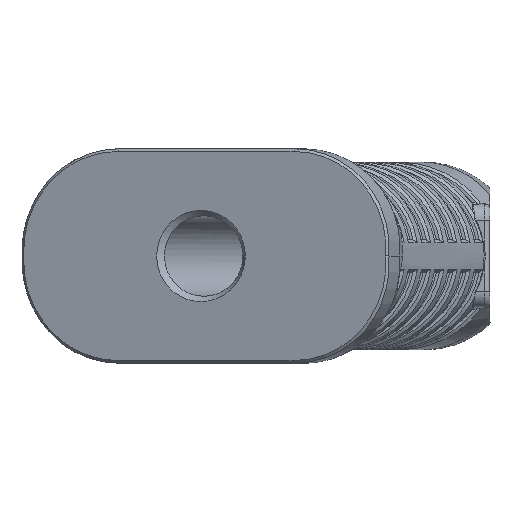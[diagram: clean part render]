
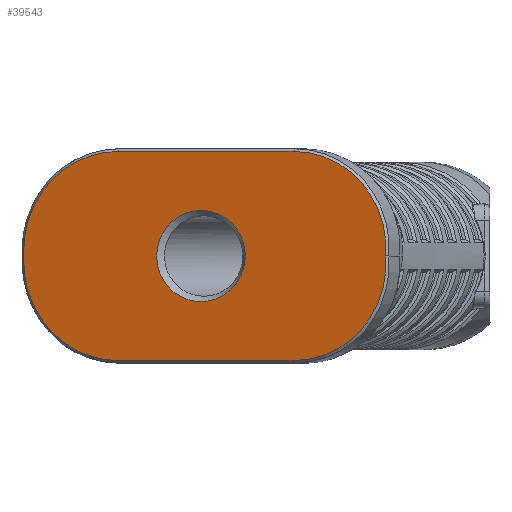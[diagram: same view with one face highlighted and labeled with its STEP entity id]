
A CAD part, front view. The second image highlights one B-rep face of the part: STEP entity #39543.
In plain terms, the highlighted planar face has unit normal (-0.307, -0.952, 0).
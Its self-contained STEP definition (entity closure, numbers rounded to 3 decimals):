
#153 = CARTESIAN_POINT ( 'NONE',  ( -220.334, -103.035, 0. ) ) ;
#214 = CARTESIAN_POINT ( 'NONE',  ( -220.334, -103.035, 4.858 ) ) ;
#435 = CARTESIAN_POINT ( 'NONE',  ( -169.904, -119.324, 2.5 ) ) ;
#636 = AXIS2_PLACEMENT_3D ( 'NONE', #8100, #1470, #26456 ) ;
#975 = VERTEX_POINT ( 'NONE', #10771 ) ;
#1265 = DIRECTION ( 'NONE',  ( -0.952, 0.307, 0. ) ) ;
#1470 = DIRECTION ( 'NONE',  ( 0.307, 0.952, 0. ) ) ;
#2087 = PLANE ( 'NONE',  #22072 ) ;
#2215 = CARTESIAN_POINT ( 'NONE',  ( -184.975, -114.456, 1. ) ) ;
#2891 = ORIENTED_EDGE ( 'NONE', *, *, #38587, .F. ) ;
#3178 = CARTESIAN_POINT ( 'NONE',  ( -217.258, -104.029, 12.827 ) ) ;
#3328 = CARTESIAN_POINT ( 'NONE',  ( -219.695, -103.242, 7.717 ) ) ;
#3631 = CARTESIAN_POINT ( 'NONE',  ( -185.365, -114.33, -7.569 ) ) ;
#4032 = CARTESIAN_POINT ( 'NONE',  ( -182.305, -115.318, 8.167 ) ) ;
#4284 = CARTESIAN_POINT ( 'NONE',  ( -213.297, -105.308, -14.8 ) ) ;
#4331 = ORIENTED_EDGE ( 'NONE', *, *, #37915, .F. ) ;
#4962 = DIRECTION ( 'NONE',  ( 0.952, -0.307, 0. ) ) ;
#5083 = CARTESIAN_POINT ( 'NONE',  ( -220.334, -103.035, 2. ) ) ;
#5459 = CARTESIAN_POINT ( 'NONE',  ( -220.334, -103.035, 0.5 ) ) ;
#5884 = CARTESIAN_POINT ( 'NONE',  ( -220.334, -103.035, 2. ) ) ;
#5949 = CARTESIAN_POINT ( 'NONE',  ( -202.734, -108.72, 20.5 ) ) ;
#6022 = CARTESIAN_POINT ( 'NONE',  ( -213.297, -105.308, 16.8 ) ) ;
#6035 = DIRECTION ( 'NONE',  ( 0.307, 0.952, 0. ) ) ;
#6374 = CARTESIAN_POINT ( 'NONE',  ( -215.784, -104.505, -12.839 ) ) ;
#6432 = CARTESIAN_POINT ( 'NONE',  ( -215.474, -104.605, 15.085 ) ) ;
#6771 = CARTESIAN_POINT ( 'NONE',  ( -195.511, -111.053, 1. ) ) ;
#6895 = CARTESIAN_POINT ( 'NONE',  ( -192.57, -112.003, -5.881 ) ) ;
#7104 = B_SPLINE_CURVE_WITH_KNOTS ( 'NONE', 3,
 ( #5884, #214, #3328, #3178, #6432, #6022 ),
 .UNSPECIFIED., .F., .F.,
 ( 4, 2, 4 ),
 ( 0., 0.5, 1. ),
 .UNSPECIFIED. ) ;
#7576 = CARTESIAN_POINT ( 'NONE',  ( -169.904, -119.324, -18.5 ) ) ;
#8100 = CARTESIAN_POINT ( 'NONE',  ( -202.734, -108.72, 2. ) ) ;
#8741 = DIRECTION ( 'NONE',  ( 0.307, 0.952, 0. ) ) ;
#8878 = DIRECTION ( 'NONE',  ( 0., 0., 1. ) ) ;
#8992 = ORIENTED_EDGE ( 'NONE', *, *, #36398, .F. ) ;
#9254 = CARTESIAN_POINT ( 'NONE',  ( -213.297, -105.308, -14.8 ) ) ;
#9646 = CIRCLE ( 'NONE', #25134, 18. ) ;
#9934 = ORIENTED_EDGE ( 'NONE', *, *, #34182, .F. ) ;
#10771 = CARTESIAN_POINT ( 'NONE',  ( -213.297, -105.308, 16.8 ) ) ;
#10776 = EDGE_CURVE ( 'NONE', #13838, #22370, #25297, .T. ) ;
#12434 = DIRECTION ( 'NONE',  ( 0.307, 0.952, 0. ) ) ;
#12942 = ORIENTED_EDGE ( 'NONE', *, *, #29042, .F. ) ;
#12952 = CARTESIAN_POINT ( 'NONE',  ( -189.153, -113.107, 9.57 ) ) ;
#13095 = CARTESIAN_POINT ( 'NONE',  ( -194.944, -111.236, 4.824 ) ) ;
#13231 = CARTESIAN_POINT ( 'NONE',  ( -195.511, -111.053, -0.275 ) ) ;
#13556 = CARTESIAN_POINT ( 'NONE',  ( -181.484, -115.583, -18.5 ) ) ;
#13838 = VERTEX_POINT ( 'NONE', #7576 ) ;
#14761 = CARTESIAN_POINT ( 'NONE',  ( -169.904, -119.324, -0.5 ) ) ;
#14790 = CARTESIAN_POINT ( 'NONE',  ( -152.835, -124.837, 1. ) ) ;
#15306 = ORIENTED_EDGE ( 'NONE', *, *, #24741, .F. ) ;
#15892 = EDGE_CURVE ( 'NONE', #22370, #22952, #15933, .T. ) ;
#15933 = CIRCLE ( 'NONE', #23954, 18.5 ) ;
#15948 = CIRCLE ( 'NONE', #30417, 18. ) ;
#16083 = CARTESIAN_POINT ( 'NONE',  ( -192.571, -112.002, 7.879 ) ) ;
#16265 = VERTEX_POINT ( 'NONE', #38779 ) ;
#16351 = CARTESIAN_POINT ( 'NONE',  ( -189.154, -113.106, -7.57 ) ) ;
#16492 = ORIENTED_EDGE ( 'NONE', *, *, #32804, .F. ) ;
#16536 = VERTEX_POINT ( 'NONE', #32579 ) ;
#17001 = VECTOR ( 'NONE', #1265, 1000. ) ;
#17911 = ORIENTED_EDGE ( 'NONE', *, *, #30891, .F. ) ;
#18851 = EDGE_LOOP ( 'NONE', ( #27252, #16492, #12942, #4331, #8992, #17911, #9934, #15306, #18893 ) ) ;
#18893 = ORIENTED_EDGE ( 'NONE', *, *, #15892, .F. ) ;
#19223 = VECTOR ( 'NONE', #4962, 1000. ) ;
#20984 = CARTESIAN_POINT ( 'NONE',  ( -202.734, -108.72, -18.5 ) ) ;
#21031 = DIRECTION ( 'NONE',  ( 0.307, 0.952, 0. ) ) ;
#21218 = DIRECTION ( 'NONE',  ( -0.673, 0.217, -0.707 ) ) ;
#21406 = VERTEX_POINT ( 'NONE', #5083 ) ;
#22013 = VERTEX_POINT ( 'NONE', #5949 ) ;
#22072 = AXIS2_PLACEMENT_3D ( 'NONE', #2215, #8741, #39977 ) ;
#22344 = CARTESIAN_POINT ( 'NONE',  ( -195.511, -111.053, 2.274 ) ) ;
#22370 = VERTEX_POINT ( 'NONE', #20984 ) ;
#22952 = VERTEX_POINT ( 'NONE', #4284 ) ;
#23568 = CARTESIAN_POINT ( 'NONE',  ( -181.484, -115.583, 20.5 ) ) ;
#23954 = AXIS2_PLACEMENT_3D ( 'NONE', #30818, #6035, #21218 ) ;
#24741 = EDGE_CURVE ( 'NONE', #22952, #31185, #39537, .T. ) ;
#25134 = AXIS2_PLACEMENT_3D ( 'NONE', #435, #12434, #37482 ) ;
#25297 = LINE ( 'NONE', #13556, #17001 ) ;
#25344 = FACE_BOUND ( 'NONE', #26550, .T. ) ;
#25377 = CARTESIAN_POINT ( 'NONE',  ( -179.306, -116.287, -2.484 ) ) ;
#25642 = CARTESIAN_POINT ( 'NONE',  ( -195.511, -111.053, 1. ) ) ;
#25681 = B_SPLINE_CURVE_WITH_KNOTS ( 'NONE', 3,
 ( #25642, #13231, #28655, #6895, #16351, #3631, #31686, #25377, #25785, #28943, #4032, #38281, #12952, #16083, #13095, #22344, #6771 ),
 .UNSPECIFIED., .T., .F.,
 ( 4, 1, 1, 1, 1, 1, 1, 1, 1, 1, 1, 1, 1, 1, 4 ),
 ( -3.142, -2.693, -2.244, -1.795, -1.346, -0.898, -0.449, 0.15, 0.449, 1.047, 1.346, 1.795, 2.244, 2.693, 3.142 ),
 .UNSPECIFIED. ) ;
#25785 = CARTESIAN_POINT ( 'NONE',  ( -178.727, -116.474, 1.467 ) ) ;
#26456 = DIRECTION ( 'NONE',  ( -0.673, 0.217, 0.707 ) ) ;
#26550 = EDGE_LOOP ( 'NONE', ( #2891 ) ) ;
#27252 = ORIENTED_EDGE ( 'NONE', *, *, #10776, .F. ) ;
#28655 = CARTESIAN_POINT ( 'NONE',  ( -194.945, -111.236, -2.824 ) ) ;
#28943 = CARTESIAN_POINT ( 'NONE',  ( -179.963, -116.075, 5.579 ) ) ;
#29042 = EDGE_CURVE ( 'NONE', #16265, #36928, #9646, .T. ) ;
#30417 = AXIS2_PLACEMENT_3D ( 'NONE', #14761, #21031, #37087 ) ;
#30818 = CARTESIAN_POINT ( 'NONE',  ( -202.734, -108.72, 0. ) ) ;
#30891 = EDGE_CURVE ( 'NONE', #21406, #975, #7104, .T. ) ;
#31185 = VERTEX_POINT ( 'NONE', #33914 ) ;
#31686 = CARTESIAN_POINT ( 'NONE',  ( -181.952, -115.432, -5.88 ) ) ;
#32433 = LINE ( 'NONE', #23568, #19223 ) ;
#32579 = CARTESIAN_POINT ( 'NONE',  ( -179.01, -116.383, 1. ) ) ;
#32804 = EDGE_CURVE ( 'NONE', #36928, #13838, #15948, .T. ) ;
#33914 = CARTESIAN_POINT ( 'NONE',  ( -220.334, -103.035, 0. ) ) ;
#34182 = EDGE_CURVE ( 'NONE', #31185, #21406, #37488, .T. ) ;
#34442 = CARTESIAN_POINT ( 'NONE',  ( -220.334, -103.035, -2.45 ) ) ;
#34674 = FACE_OUTER_BOUND ( 'NONE', #18851, .T. ) ;
#35042 = VECTOR ( 'NONE', #8878, 1000. ) ;
#36398 = EDGE_CURVE ( 'NONE', #975, #22013, #39830, .T. ) ;
#36928 = VERTEX_POINT ( 'NONE', #14790 ) ;
#37087 = DIRECTION ( 'NONE',  ( 0.673, -0.217, -0.707 ) ) ;
#37482 = DIRECTION ( 'NONE',  ( 0.673, -0.217, 0.707 ) ) ;
#37488 = LINE ( 'NONE', #5459, #35042 ) ;
#37915 = EDGE_CURVE ( 'NONE', #22013, #16265, #32433, .T. ) ;
#38018 = CARTESIAN_POINT ( 'NONE',  ( -219.242, -103.388, -8.168 ) ) ;
#38281 = CARTESIAN_POINT ( 'NONE',  ( -185.79, -114.193, 9.568 ) ) ;
#38587 = EDGE_CURVE ( 'NONE', #16536, #16536, #25681, .T. ) ;
#38779 = CARTESIAN_POINT ( 'NONE',  ( -169.904, -119.324, 20.5 ) ) ;
#39537 = B_SPLINE_CURVE_WITH_KNOTS ( 'NONE', 3,
 ( #9254, #6374, #38018, #34442, #153 ),
 .UNSPECIFIED., .F., .F.,
 ( 4, 1, 4 ),
 ( 0., 0.571, 1. ),
 .UNSPECIFIED. ) ;
#39543 = ADVANCED_FACE ( 'NONE', ( #34674, #25344 ), #2087, .F. ) ;
#39830 = CIRCLE ( 'NONE', #636, 18.5 ) ;
#39977 = DIRECTION ( 'NONE',  ( -0.906, 0.292, -0.307 ) ) ;
